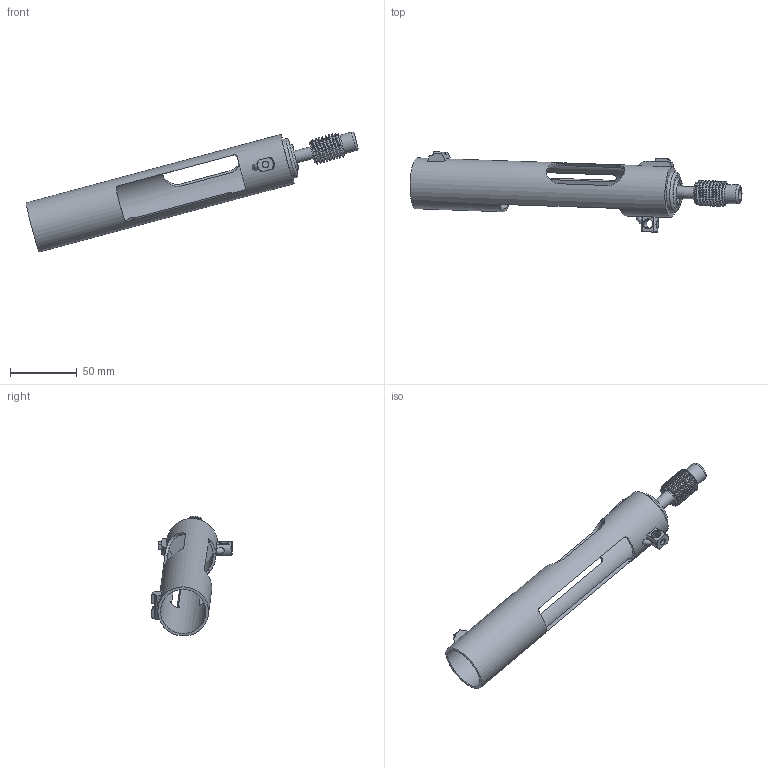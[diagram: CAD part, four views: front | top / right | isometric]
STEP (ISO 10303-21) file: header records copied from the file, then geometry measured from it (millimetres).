
FILE_DESCRIPTION(/* description */ (''),/* implementation_level */ '2;1');
FILE_NAME(/* name */ 'KG99mini v1.step',/* time_stamp */ '2025-06-02T16:12:34-07:00',/* author */ (''),/* organization */ (''),/* preprocessor_version */ 'ST-DEVELOPER v20.1',/* originating_system */ 'Autodesk Translation Framework v14.10.0.0',/* authorisation */ '');
FILE_SCHEMA (('AUTOMOTIVE_DESIGN { 1 0 10303 214 3 1 1 }'));
Length unit declared in the file: millimetre
Products named in the file (1): KG99mini
Bounding box: 248.49 x 60.24 x 89.8 mm (x, y, z)
Volume: 53177.6 mm3; surface area: 46421.6 mm2
Topology: 4 solids, 4 shells, 112 faces, 316 edges, 217 vertices
Faces by surface type: cylinder 52, plane 42, cone 7, bspline 6, torus 5
Full cylindrical faces by diameter (mm): 5 x2, 5.5 x1, 7 x1, 8 x1, 9 x2, 14.2 x1, 16.025 x8, 18.885 x8, 34.1 x1, 38.1 x1
Entity records: 14272 total; most frequent: CARTESIAN_POINT 11441, ORIENTED_EDGE 632, DIRECTION 501, EDGE_CURVE 316, VERTEX_POINT 217, AXIS2_PLACEMENT_3D 187, EDGE_LOOP 131, LINE 127
